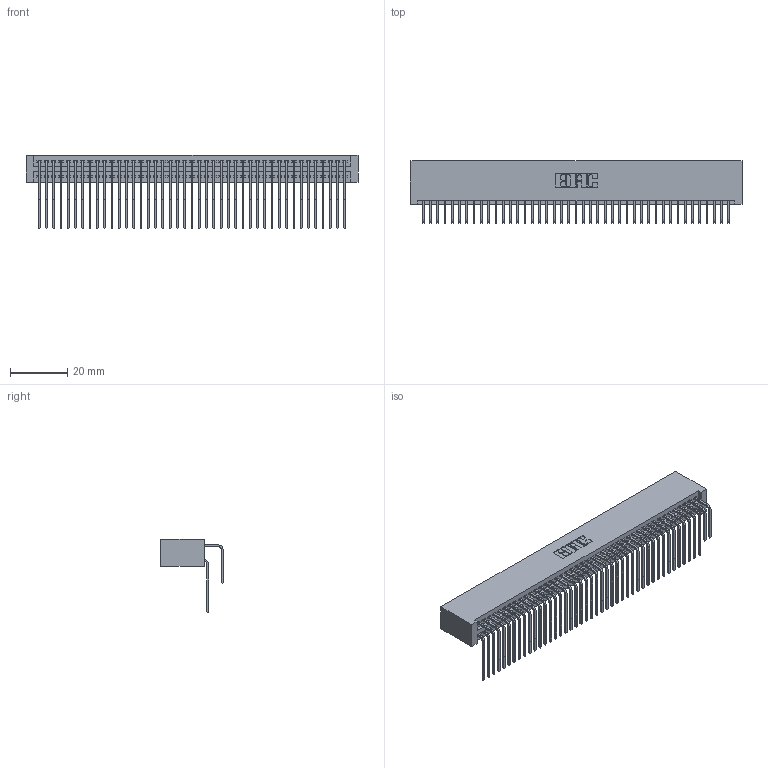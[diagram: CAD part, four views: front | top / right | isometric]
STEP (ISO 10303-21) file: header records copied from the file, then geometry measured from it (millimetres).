
FILE_DESCRIPTION (( 'STEP AP203' ), '1' );
FILE_NAME ('395-086-558-201.STEP', '2018-11-28T22:09:12', ( '' ), ( '' ), 'SwSTEP 2.0', 'SolidWorks 2016', '' );
FILE_SCHEMA (( 'CONFIG_CONTROL_DESIGN' ));
Length unit declared in the file: inch
Products named in the file (4): 345-292-001_558 559 Tail - 1; 345-292-001_558 Tail - 2; 395-086-558-201; 345 Part_No Mounting Lugs
Assembly tree (87 placements, depth 2):
  395-086-558-201
    345 Part_No Mounting Lugs
    345-292-001_558 559 Tail - 1  x43
    345-292-001_558 Tail - 2  x43
Bounding box: 115.82 x 21.83 x 25.53 mm (x, y, z)
Volume: 12372.6 mm3; surface area: 20944.2 mm2
Topology: 87 solids, 87 shells, 4590 faces, 13647 edges, 8982 vertices
Faces by surface type: plane 3086, cylinder 1504
Entity records: 34979 total; most frequent: CARTESIAN_POINT 5907, ORIENTED_EDGE 5790, DIRECTION 5175, EDGE_CURVE 2895, VECTOR 2559, LINE 2559, VERTEX_POINT 1926, AXIS2_PLACEMENT_3D 1308
